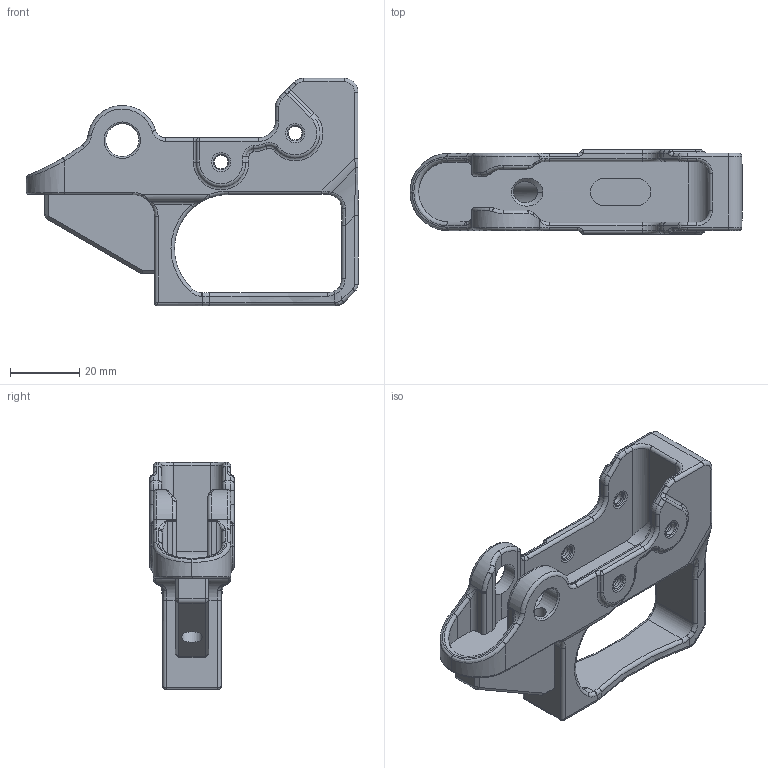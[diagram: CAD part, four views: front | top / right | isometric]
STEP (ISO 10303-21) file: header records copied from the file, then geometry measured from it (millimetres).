
FILE_DESCRIPTION(/* description */ (''),/* implementation_level */ '2;1');
FILE_NAME(/* name */ 'Trigger Test Jig V1.5 v1.step',/* time_stamp */ '2021-04-08T20:13:29-04:00',/* author */ (''),/* organization */ (''),/* preprocessor_version */ 'ST-DEVELOPER v18.1',/* originating_system */ 'Autodesk Translation Framework v10.6.0.1341',/* authorisation */ '');
FILE_SCHEMA (('AUTOMOTIVE_DESIGN { 1 0 10303 214 3 1 1 }'));
Length unit declared in the file: millimetre
Products named in the file (1): Trigger Test Jig V1.5
Bounding box: 95.95 x 24.33 x 65.72 mm (x, y, z)
Volume: 33005.3 mm3; surface area: 18045.7 mm2
Topology: 1 solids, 1 shells, 409 faces, 1005 edges, 585 vertices
Faces by surface type: cylinder 148, torus 109, bspline 73, plane 58, cone 15, sphere 6
Full cylindrical faces by diameter (mm): 3.962 x4, 4 x4, 6.097 x1, 9.55 x2
Entity records: 14226 total; most frequent: CARTESIAN_POINT 4701, DIRECTION 2054, ORIENTED_EDGE 1994, EDGE_CURVE 997, AXIS2_PLACEMENT_3D 866, VERTEX_POINT 585, CIRCLE 493, EDGE_LOOP 424
